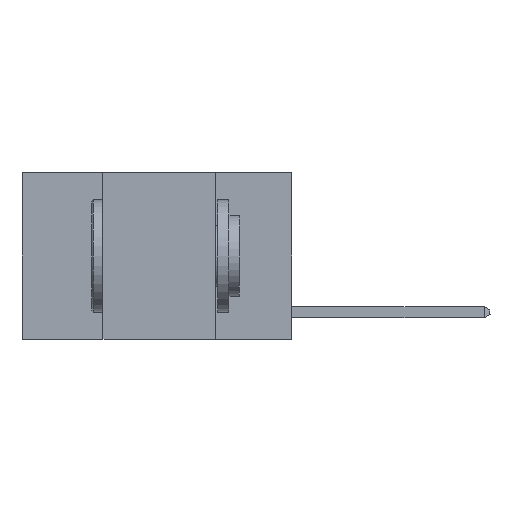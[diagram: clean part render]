
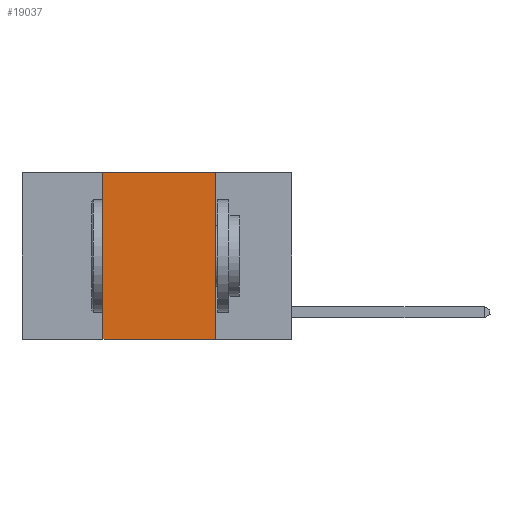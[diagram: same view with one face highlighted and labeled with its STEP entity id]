
A CAD part, left-side view. The second image highlights one B-rep face of the part: STEP entity #19037.
In plain terms, the highlighted planar face has unit normal (-1, 0, 0).
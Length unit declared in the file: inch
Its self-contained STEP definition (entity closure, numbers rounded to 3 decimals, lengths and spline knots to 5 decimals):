
#65 = CARTESIAN_POINT ( 'NONE',  ( 0., 0.6, 0. ) ) ;
#146 = CARTESIAN_POINT ( 'NONE',  ( 0., 0.6, 0. ) ) ;
#2022 = DIRECTION ( 'NONE',  ( 0., 0., -1. ) ) ;
#2668 = CARTESIAN_POINT ( 'NONE',  ( 0., 0.17, 0. ) ) ;
#3127 = VERTEX_POINT ( 'NONE', #14304 ) ;
#3598 = EDGE_CURVE ( 'NONE', #23660, #22961, #17015, .T. ) ;
#3786 = VECTOR ( 'NONE', #19725, 39.37008 ) ;
#3815 = EDGE_CURVE ( 'NONE', #16423, #23660, #9490, .T. ) ;
#4138 = VECTOR ( 'NONE', #15143, 39.37008 ) ;
#4495 = EDGE_CURVE ( 'NONE', #22961, #3127, #19838, .T. ) ;
#5343 = VECTOR ( 'NONE', #11251, 39.37008 ) ;
#5582 = ORIENTED_EDGE ( 'NONE', *, *, #3598, .F. ) ;
#6996 = LINE ( 'NONE', #12677, #19764 ) ;
#7918 = FACE_OUTER_BOUND ( 'NONE', #17415, .T. ) ;
#9490 = LINE ( 'NONE', #23777, #5343 ) ;
#10953 = AXIS2_PLACEMENT_3D ( 'NONE', #65, #20932, #2022 ) ;
#11251 = DIRECTION ( 'NONE',  ( 0., 0., 1. ) ) ;
#12072 = ORIENTED_EDGE ( 'NONE', *, *, #15986, .T. ) ;
#12677 = CARTESIAN_POINT ( 'NONE',  ( 0., 0.6, -0.37 ) ) ;
#14304 = CARTESIAN_POINT ( 'NONE',  ( 0., 0.17, -0.37 ) ) ;
#14781 = ORIENTED_EDGE ( 'NONE', *, *, #4495, .F. ) ;
#15143 = DIRECTION ( 'NONE',  ( 0., -1., 0. ) ) ;
#15986 = EDGE_CURVE ( 'NONE', #16423, #3127, #6996, .T. ) ;
#16423 = VERTEX_POINT ( 'NONE', #22543 ) ;
#17015 = LINE ( 'NONE', #146, #4138 ) ;
#17415 = EDGE_LOOP ( 'NONE', ( #14781, #5582, #21040, #12072 ) ) ;
#18115 = CARTESIAN_POINT ( 'NONE',  ( 0., 0.17, 0. ) ) ;
#18868 = DIRECTION ( 'NONE',  ( 0., -1., 0. ) ) ;
#19037 = ADVANCED_FACE ( 'NONE', ( #7918 ), #19194, .F. ) ;
#19045 = CARTESIAN_POINT ( 'NONE',  ( 0., 0.42, 0. ) ) ;
#19194 = PLANE ( 'NONE',  #10953 ) ;
#19725 = DIRECTION ( 'NONE',  ( 0., 0., -1. ) ) ;
#19764 = VECTOR ( 'NONE', #18868, 39.37008 ) ;
#19838 = LINE ( 'NONE', #2668, #3786 ) ;
#20932 = DIRECTION ( 'NONE',  ( 1., 0., 0. ) ) ;
#21040 = ORIENTED_EDGE ( 'NONE', *, *, #3815, .F. ) ;
#22543 = CARTESIAN_POINT ( 'NONE',  ( 0., 0.42, -0.37 ) ) ;
#22961 = VERTEX_POINT ( 'NONE', #18115 ) ;
#23660 = VERTEX_POINT ( 'NONE', #19045 ) ;
#23777 = CARTESIAN_POINT ( 'NONE',  ( 0., 0.42, 0. ) ) ;
